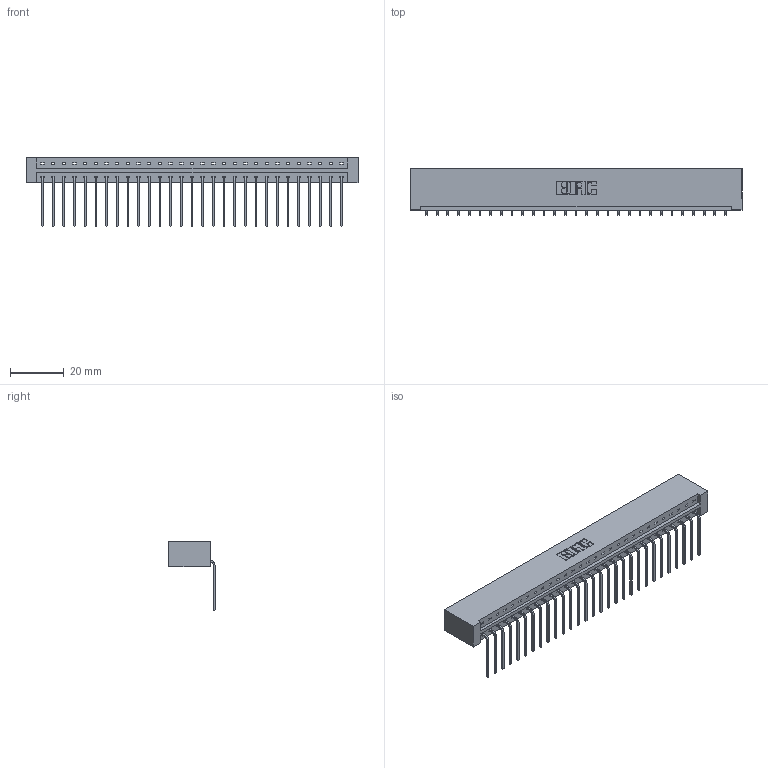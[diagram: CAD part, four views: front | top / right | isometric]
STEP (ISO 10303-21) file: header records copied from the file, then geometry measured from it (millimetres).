
FILE_DESCRIPTION (( 'STEP AP203' ), '1' );
FILE_NAME ('833-029-559-101.STEP', '2020-06-02T11:31:32', ( '' ), ( '' ), 'SwSTEP 2.0', 'SolidWorks 2020', '' );
FILE_SCHEMA (( 'CONFIG_CONTROL_DESIGN' ));
Length unit declared in the file: inch
Products named in the file (3): 833-029-559-101; 345-292-001_558 559 Tail - 1; 833 Part_Lugless
Assembly tree (30 placements, depth 2):
  833-029-559-101
    833 Part_Lugless
    345-292-001_558 559 Tail - 1  x29
Bounding box: 123.16 x 17.09 x 25.53 mm (x, y, z)
Volume: 12991.4 mm3; surface area: 14520.4 mm2
Topology: 30 solids, 30 shells, 1846 faces, 5565 edges, 3670 vertices
Faces by surface type: plane 1342, cylinder 504
Entity records: 19217 total; most frequent: CARTESIAN_POINT 3325, ORIENTED_EDGE 3290, DIRECTION 2823, EDGE_CURVE 1645, VECTOR 1525, LINE 1525, VERTEX_POINT 1094, AXIS2_PLACEMENT_3D 649
